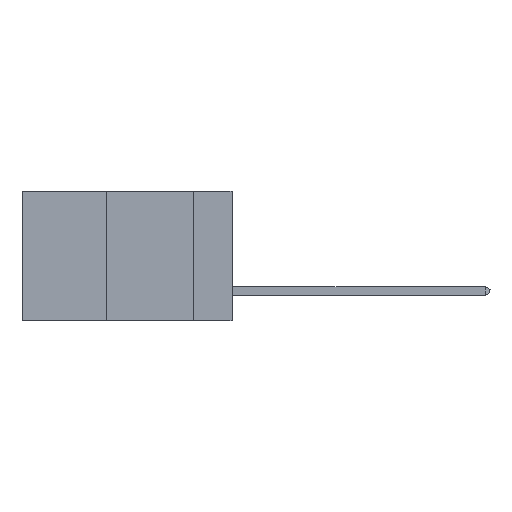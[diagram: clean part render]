
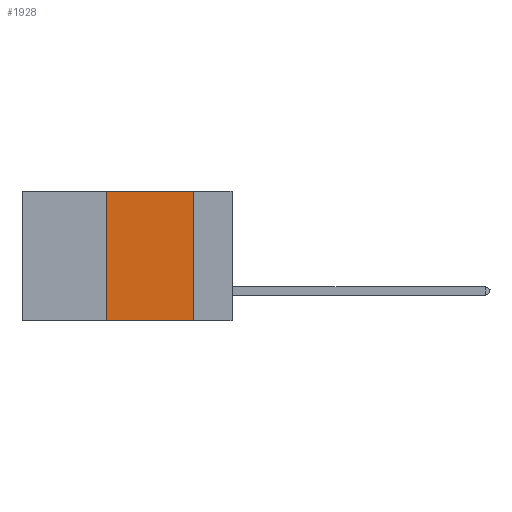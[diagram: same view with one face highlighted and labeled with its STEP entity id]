
A CAD part, left-side view. The second image highlights one B-rep face of the part: STEP entity #1928.
In plain terms, the highlighted planar face has unit normal (-1, 0, 0).
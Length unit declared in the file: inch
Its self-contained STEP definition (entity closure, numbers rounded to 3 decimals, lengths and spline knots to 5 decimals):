
#401 = DIRECTION ( 'NONE',  ( 1., 0., 0. ) ) ;
#740 = DIRECTION ( 'NONE',  ( 0., 0., 1. ) ) ;
#993 = VECTOR ( 'NONE', #27235, 39.37008 ) ;
#1119 = CARTESIAN_POINT ( 'NONE',  ( 0., 0.11, 0. ) ) ;
#1283 = EDGE_CURVE ( 'NONE', #21865, #27339, #7346, .T. ) ;
#1464 = ORIENTED_EDGE ( 'NONE', *, *, #15325, .F. ) ;
#1928 = ADVANCED_FACE ( 'NONE', ( #20059 ), #4737, .F. ) ;
#4457 = ORIENTED_EDGE ( 'NONE', *, *, #1283, .F. ) ;
#4737 = PLANE ( 'NONE',  #23559 ) ;
#4814 = CARTESIAN_POINT ( 'NONE',  ( 0., 0.36, -0.37 ) ) ;
#4856 = LINE ( 'NONE', #20856, #5214 ) ;
#5214 = VECTOR ( 'NONE', #740, 39.37008 ) ;
#6557 = CARTESIAN_POINT ( 'NONE',  ( 0., 0.11, -0.37 ) ) ;
#6933 = CARTESIAN_POINT ( 'NONE',  ( 0., 0.6, 0. ) ) ;
#7346 = LINE ( 'NONE', #17844, #22497 ) ;
#8692 = DIRECTION ( 'NONE',  ( 0., 0., -1. ) ) ;
#9938 = LINE ( 'NONE', #20472, #993 ) ;
#10890 = DIRECTION ( 'NONE',  ( 0., 0., -1. ) ) ;
#11154 = DIRECTION ( 'NONE',  ( 0., -1., 0. ) ) ;
#12750 = CARTESIAN_POINT ( 'NONE',  ( 0., 0.36, 0. ) ) ;
#13829 = CARTESIAN_POINT ( 'NONE',  ( 0., 0.11, 0. ) ) ;
#14352 = VECTOR ( 'NONE', #8692, 39.37008 ) ;
#15325 = EDGE_CURVE ( 'NONE', #22799, #21865, #4856, .T. ) ;
#16748 = EDGE_CURVE ( 'NONE', #22799, #28334, #9938, .T. ) ;
#17507 = EDGE_LOOP ( 'NONE', ( #20184, #4457, #1464, #18448 ) ) ;
#17753 = EDGE_CURVE ( 'NONE', #27339, #28334, #22566, .T. ) ;
#17844 = CARTESIAN_POINT ( 'NONE',  ( 0., 0.6, 0. ) ) ;
#18448 = ORIENTED_EDGE ( 'NONE', *, *, #16748, .T. ) ;
#20059 = FACE_OUTER_BOUND ( 'NONE', #17507, .T. ) ;
#20184 = ORIENTED_EDGE ( 'NONE', *, *, #17753, .F. ) ;
#20472 = CARTESIAN_POINT ( 'NONE',  ( 0., 0.6, -0.37 ) ) ;
#20856 = CARTESIAN_POINT ( 'NONE',  ( 0., 0.36, 0. ) ) ;
#21865 = VERTEX_POINT ( 'NONE', #12750 ) ;
#22497 = VECTOR ( 'NONE', #11154, 39.37008 ) ;
#22566 = LINE ( 'NONE', #1119, #14352 ) ;
#22799 = VERTEX_POINT ( 'NONE', #4814 ) ;
#23559 = AXIS2_PLACEMENT_3D ( 'NONE', #6933, #401, #10890 ) ;
#27235 = DIRECTION ( 'NONE',  ( 0., -1., 0. ) ) ;
#27339 = VERTEX_POINT ( 'NONE', #13829 ) ;
#28334 = VERTEX_POINT ( 'NONE', #6557 ) ;
